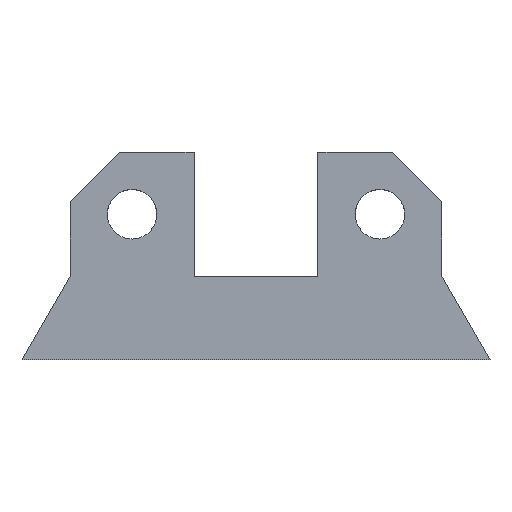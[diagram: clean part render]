
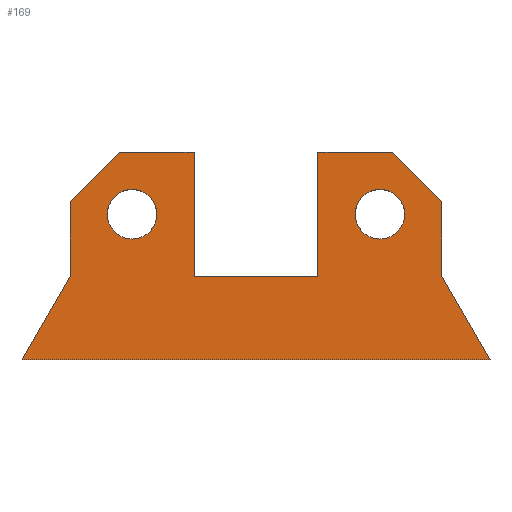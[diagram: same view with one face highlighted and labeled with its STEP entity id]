
A CAD part, top view. The second image highlights one B-rep face of the part: STEP entity #169.
In plain terms, the highlighted planar face has unit normal (0, 0, 1).
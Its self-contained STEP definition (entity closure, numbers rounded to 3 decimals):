
#7 = VECTOR ( 'NONE', #51, 1000. ) ;
#9 = DIRECTION ( 'NONE',  ( -0.707, 0.707, 0. ) ) ;
#13 = ORIENTED_EDGE ( 'NONE', *, *, #546, .F. ) ;
#15 = VERTEX_POINT ( 'NONE', #151 ) ;
#18 = DIRECTION ( 'NONE',  ( 1., 0., 0. ) ) ;
#21 = CARTESIAN_POINT ( 'NONE',  ( 10., 38.292, 5. ) ) ;
#26 = VERTEX_POINT ( 'NONE', #156 ) ;
#29 = ORIENTED_EDGE ( 'NONE', *, *, #577, .F. ) ;
#37 = LINE ( 'NONE', #560, #145 ) ;
#40 = DIRECTION ( 'NONE',  ( -0.5, -0.866, 0. ) ) ;
#44 = VECTOR ( 'NONE', #40, 1000. ) ;
#51 = DIRECTION ( 'NONE',  ( 0., 1., 0. ) ) ;
#54 = DIRECTION ( 'NONE',  ( 1., 0., 0. ) ) ;
#64 = VERTEX_POINT ( 'NONE', #311 ) ;
#66 = VERTEX_POINT ( 'NONE', #279 ) ;
#71 = CARTESIAN_POINT ( 'NONE',  ( 2.5, 35.792, 5. ) ) ;
#73 = VECTOR ( 'NONE', #492, 1000. ) ;
#83 = VERTEX_POINT ( 'NONE', #192 ) ;
#87 = DIRECTION ( 'NONE',  ( 0., 0., 1. ) ) ;
#89 = CARTESIAN_POINT ( 'NONE',  ( 7.5, 35.792, 5. ) ) ;
#98 = VERTEX_POINT ( 'NONE', #317 ) ;
#100 = CARTESIAN_POINT ( 'NONE',  ( 25.646, 25.646, 5. ) ) ;
#104 = ORIENTED_EDGE ( 'NONE', *, *, #549, .F. ) ;
#107 = CARTESIAN_POINT ( 'NONE',  ( -2.5, 35.792, 5. ) ) ;
#110 = DIRECTION ( 'NONE',  ( 1., 0., 0. ) ) ;
#117 = CARTESIAN_POINT ( 'NONE',  ( 0., 38.292, 5. ) ) ;
#124 = EDGE_LOOP ( 'NONE', ( #140, #130 ) ) ;
#130 = ORIENTED_EDGE ( 'NONE', *, *, #555, .F. ) ;
#139 = VERTEX_POINT ( 'NONE', #599 ) ;
#140 = ORIENTED_EDGE ( 'NONE', *, *, #515, .F. ) ;
#141 = CARTESIAN_POINT ( 'NONE',  ( -2.5, 35.792, 5. ) ) ;
#142 = EDGE_LOOP ( 'NONE', ( #224, #13 ) ) ;
#143 = VERTEX_POINT ( 'NONE', #327 ) ;
#145 = VECTOR ( 'NONE', #346, 1000. ) ;
#146 = FACE_OUTER_BOUND ( 'NONE', #217, .T. ) ;
#147 = CARTESIAN_POINT ( 'NONE',  ( 7.5, 35.792, 5. ) ) ;
#149 = CARTESIAN_POINT ( 'NONE',  ( 14.442, 32.429, 5. ) ) ;
#151 = CARTESIAN_POINT ( 'NONE',  ( 11., 38.292, 5. ) ) ;
#156 = CARTESIAN_POINT ( 'NONE',  ( 1., 38.292, 5. ) ) ;
#159 = VECTOR ( 'NONE', #227, 1000. ) ;
#160 = DIRECTION ( 'NONE',  ( 0., 0., 1. ) ) ;
#166 = CARTESIAN_POINT ( 'NONE',  ( 12.5, 35.792, 5. ) ) ;
#167 = CIRCLE ( 'NONE', #425, 1. ) ;
#169 = ADVANCED_FACE ( 'NONE', ( #420, #222, #146 ), #329, .T. ) ;
#172 = DIRECTION ( 'NONE',  ( 1., 0., 0. ) ) ;
#173 = CARTESIAN_POINT ( 'NONE',  ( -0.5, 40.792, 5. ) ) ;
#175 = CARTESIAN_POINT ( 'NONE',  ( -20.646, 20.646, 5. ) ) ;
#180 = VECTOR ( 'NONE', #18, 1000. ) ;
#182 = VECTOR ( 'NONE', #278, 1000. ) ;
#189 = DIRECTION ( 'NONE',  ( 1., 0., 0. ) ) ;
#192 = CARTESIAN_POINT ( 'NONE',  ( 10.5, 40.792, 5. ) ) ;
#194 = DIRECTION ( 'NONE',  ( 1., 0., 0. ) ) ;
#196 = VECTOR ( 'NONE', #337, 1000. ) ;
#217 = EDGE_LOOP ( 'NONE', ( #482, #530, #29, #366, #292, #510, #484, #481, #587, #277, #104, #542 ) ) ;
#222 = FACE_BOUND ( 'NONE', #142, .T. ) ;
#224 = ORIENTED_EDGE ( 'NONE', *, *, #529, .F. ) ;
#227 = DIRECTION ( 'NONE',  ( -0.5, 0.866, 0. ) ) ;
#232 = CARTESIAN_POINT ( 'NONE',  ( -4.442, 32.429, 5. ) ) ;
#238 = VERTEX_POINT ( 'NONE', #89 ) ;
#244 = VERTEX_POINT ( 'NONE', #166 ) ;
#249 = DIRECTION ( 'NONE',  ( 1., 0., 0. ) ) ;
#251 = DIRECTION ( 'NONE',  ( 0., 0., 1. ) ) ;
#255 = LINE ( 'NONE', #100, #302 ) ;
#258 = CARTESIAN_POINT ( 'NONE',  ( 7.5, 40.792, 5. ) ) ;
#261 = LINE ( 'NONE', #147, #7 ) ;
#266 = VECTOR ( 'NONE', #110, 1000. ) ;
#267 = VERTEX_POINT ( 'NONE', #173 ) ;
#272 = CARTESIAN_POINT ( 'NONE',  ( -2.5, 40.792, 5. ) ) ;
#274 = CARTESIAN_POINT ( 'NONE',  ( 12.5, 40.792, 5. ) ) ;
#277 = ORIENTED_EDGE ( 'NONE', *, *, #533, .F. ) ;
#278 = DIRECTION ( 'NONE',  ( 1., 0., 0. ) ) ;
#279 = CARTESIAN_POINT ( 'NONE',  ( -2.5, 35.792, 5. ) ) ;
#290 = LINE ( 'NONE', #71, #182 ) ;
#291 = CIRCLE ( 'NONE', #435, 1. ) ;
#292 = ORIENTED_EDGE ( 'NONE', *, *, #521, .T. ) ;
#302 = VECTOR ( 'NONE', #9, 1000. ) ;
#310 = DIRECTION ( 'NONE',  ( 0., 0., 1. ) ) ;
#311 = CARTESIAN_POINT ( 'NONE',  ( -4.442, 32.429, 5. ) ) ;
#314 = CARTESIAN_POINT ( 'NONE',  ( 2.5, 35.792, 5. ) ) ;
#315 = LINE ( 'NONE', #107, #44 ) ;
#316 = VERTEX_POINT ( 'NONE', #358 ) ;
#317 = CARTESIAN_POINT ( 'NONE',  ( 7.5, 40.792, 5. ) ) ;
#327 = CARTESIAN_POINT ( 'NONE',  ( 2.5, 40.792, 5. ) ) ;
#329 = PLANE ( 'NONE',  #485 ) ;
#337 = DIRECTION ( 'NONE',  ( 1., 0., 0. ) ) ;
#342 = LINE ( 'NONE', #141, #360 ) ;
#346 = DIRECTION ( 'NONE',  ( 0., -1., 0. ) ) ;
#348 = CARTESIAN_POINT ( 'NONE',  ( 14.442, 32.429, 5. ) ) ;
#352 = VERTEX_POINT ( 'NONE', #314 ) ;
#356 = LINE ( 'NONE', #175, #73 ) ;
#357 = VERTEX_POINT ( 'NONE', #348 ) ;
#358 = CARTESIAN_POINT ( 'NONE',  ( 12.5, 38.792, 5. ) ) ;
#360 = VECTOR ( 'NONE', #476, 1000. ) ;
#365 = LINE ( 'NONE', #232, #180 ) ;
#366 = ORIENTED_EDGE ( 'NONE', *, *, #523, .T. ) ;
#371 = CARTESIAN_POINT ( 'NONE',  ( 0., 0., 5. ) ) ;
#377 = CARTESIAN_POINT ( 'NONE',  ( -1., 38.292, 5. ) ) ;
#381 = LINE ( 'NONE', #149, #159 ) ;
#393 = LINE ( 'NONE', #274, #463 ) ;
#420 = FACE_BOUND ( 'NONE', #124, .T. ) ;
#425 = AXIS2_PLACEMENT_3D ( 'NONE', #514, #583, #54 ) ;
#432 = AXIS2_PLACEMENT_3D ( 'NONE', #117, #160, #194 ) ;
#435 = AXIS2_PLACEMENT_3D ( 'NONE', #609, #87, #172 ) ;
#439 = AXIS2_PLACEMENT_3D ( 'NONE', #21, #310, #189 ) ;
#463 = VECTOR ( 'NONE', #570, 1000. ) ;
#476 = DIRECTION ( 'NONE',  ( 0., 1., 0. ) ) ;
#481 = ORIENTED_EDGE ( 'NONE', *, *, #545, .T. ) ;
#482 = ORIENTED_EDGE ( 'NONE', *, *, #520, .F. ) ;
#484 = ORIENTED_EDGE ( 'NONE', *, *, #516, .F. ) ;
#485 = AXIS2_PLACEMENT_3D ( 'NONE', #371, #251, #249 ) ;
#490 = LINE ( 'NONE', #272, #266 ) ;
#492 = DIRECTION ( 'NONE',  ( -0.707, -0.707, 0. ) ) ;
#500 = CIRCLE ( 'NONE', #439, 1. ) ;
#510 = ORIENTED_EDGE ( 'NONE', *, *, #557, .T. ) ;
#512 = CIRCLE ( 'NONE', #432, 1. ) ;
#514 = CARTESIAN_POINT ( 'NONE',  ( 10., 38.292, 5. ) ) ;
#515 = EDGE_CURVE ( 'NONE', #15, #593, #500, .T. ) ;
#516 = EDGE_CURVE ( 'NONE', #316, #244, #393, .T. ) ;
#520 = EDGE_CURVE ( 'NONE', #267, #143, #490, .T. ) ;
#521 = EDGE_CURVE ( 'NONE', #64, #357, #365, .T. ) ;
#523 = EDGE_CURVE ( 'NONE', #66, #64, #315, .T. ) ;
#529 = EDGE_CURVE ( 'NONE', #26, #610, #291, .T. ) ;
#530 = ORIENTED_EDGE ( 'NONE', *, *, #538, .T. ) ;
#533 = EDGE_CURVE ( 'NONE', #238, #98, #261, .T. ) ;
#538 = EDGE_CURVE ( 'NONE', #267, #139, #356, .T. ) ;
#542 = ORIENTED_EDGE ( 'NONE', *, *, #566, .F. ) ;
#545 = EDGE_CURVE ( 'NONE', #316, #83, #255, .T. ) ;
#546 = EDGE_CURVE ( 'NONE', #610, #26, #512, .T. ) ;
#549 = EDGE_CURVE ( 'NONE', #352, #238, #290, .T. ) ;
#555 = EDGE_CURVE ( 'NONE', #593, #15, #167, .T. ) ;
#557 = EDGE_CURVE ( 'NONE', #357, #244, #381, .T. ) ;
#560 = CARTESIAN_POINT ( 'NONE',  ( 2.5, 40.792, 5. ) ) ;
#563 = CARTESIAN_POINT ( 'NONE',  ( 9., 38.292, 5. ) ) ;
#566 = EDGE_CURVE ( 'NONE', #143, #352, #37, .T. ) ;
#570 = DIRECTION ( 'NONE',  ( 0., -1., 0. ) ) ;
#577 = EDGE_CURVE ( 'NONE', #66, #139, #342, .T. ) ;
#582 = LINE ( 'NONE', #258, #196 ) ;
#583 = DIRECTION ( 'NONE',  ( 0., 0., 1. ) ) ;
#587 = ORIENTED_EDGE ( 'NONE', *, *, #592, .F. ) ;
#592 = EDGE_CURVE ( 'NONE', #98, #83, #582, .T. ) ;
#593 = VERTEX_POINT ( 'NONE', #563 ) ;
#599 = CARTESIAN_POINT ( 'NONE',  ( -2.5, 38.792, 5. ) ) ;
#609 = CARTESIAN_POINT ( 'NONE',  ( 0., 38.292, 5. ) ) ;
#610 = VERTEX_POINT ( 'NONE', #377 ) ;
